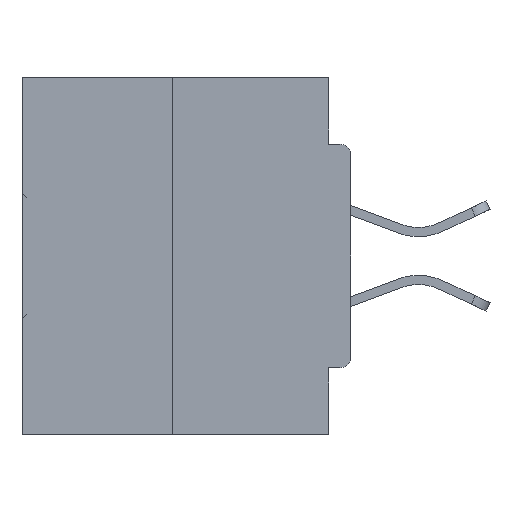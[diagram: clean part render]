
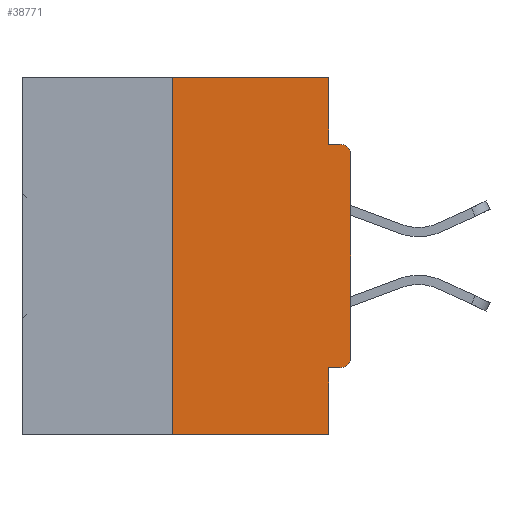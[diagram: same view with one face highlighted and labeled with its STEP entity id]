
A CAD part, left-side view. The second image highlights one B-rep face of the part: STEP entity #38771.
In plain terms, the highlighted planar face has unit normal (-1, 0, 0).
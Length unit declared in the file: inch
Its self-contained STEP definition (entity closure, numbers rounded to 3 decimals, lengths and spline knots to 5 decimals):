
#1341 = EDGE_CURVE ( 'NONE', #25626, #3799, #30260, .T. ) ;
#2344 = CARTESIAN_POINT ( 'NONE',  ( 0., 0.015, -0.4065 ) ) ;
#3655 = CIRCLE ( 'NONE', #26507, 0.015 ) ;
#3799 = VERTEX_POINT ( 'NONE', #38552 ) ;
#4048 = CARTESIAN_POINT ( 'NONE',  ( 0., 0., -0.4065 ) ) ;
#4069 = LINE ( 'NONE', #24545, #23537 ) ;
#4107 = DIRECTION ( 'NONE',  ( 0., -1., 0. ) ) ;
#4345 = DIRECTION ( 'NONE',  ( 0., 0., -1. ) ) ;
#4369 = VERTEX_POINT ( 'NONE', #11530 ) ;
#4495 = PLANE ( 'NONE',  #8993 ) ;
#4661 = DIRECTION ( 'NONE',  ( 1., 0., 0. ) ) ;
#4861 = DIRECTION ( 'NONE',  ( 0., -1., 0. ) ) ;
#5702 = LINE ( 'NONE', #25557, #31039 ) ;
#5829 = ORIENTED_EDGE ( 'NONE', *, *, #20865, .F. ) ;
#6126 = CARTESIAN_POINT ( 'NONE',  ( 0., 0.25, -0.5 ) ) ;
#6501 = VECTOR ( 'NONE', #15353, 39.37008 ) ;
#6539 = VECTOR ( 'NONE', #28233, 39.37008 ) ;
#6640 = EDGE_CURVE ( 'NONE', #15424, #7585, #7974, .T. ) ;
#7585 = VERTEX_POINT ( 'NONE', #31180 ) ;
#7686 = EDGE_CURVE ( 'NONE', #7585, #4369, #42402, .T. ) ;
#7974 = LINE ( 'NONE', #9703, #10125 ) ;
#8915 = CARTESIAN_POINT ( 'NONE',  ( 0., 0., -0.0935 ) ) ;
#8979 = ORIENTED_EDGE ( 'NONE', *, *, #30874, .T. ) ;
#8993 = AXIS2_PLACEMENT_3D ( 'NONE', #39080, #4661, #4345 ) ;
#9703 = CARTESIAN_POINT ( 'NONE',  ( 0., 0.25, 0. ) ) ;
#9841 = DIRECTION ( 'NONE',  ( 0., 0., 1. ) ) ;
#10125 = VECTOR ( 'NONE', #9841, 39.37008 ) ;
#10878 = ORIENTED_EDGE ( 'NONE', *, *, #24244, .T. ) ;
#11193 = VERTEX_POINT ( 'NONE', #11516 ) ;
#11411 = EDGE_CURVE ( 'NONE', #27176, #3799, #3655, .T. ) ;
#11516 = CARTESIAN_POINT ( 'NONE',  ( 0., 0.031, -0.5 ) ) ;
#11530 = CARTESIAN_POINT ( 'NONE',  ( 0., 0.031, 0. ) ) ;
#12800 = LINE ( 'NONE', #21237, #32812 ) ;
#13100 = DIRECTION ( 'NONE',  ( 0., 0., -1. ) ) ;
#14844 = DIRECTION ( 'NONE',  ( -1., 0., 0. ) ) ;
#14949 = ORIENTED_EDGE ( 'NONE', *, *, #30938, .F. ) ;
#15353 = DIRECTION ( 'NONE',  ( 0., 0., 1. ) ) ;
#15424 = VERTEX_POINT ( 'NONE', #6126 ) ;
#16088 = CARTESIAN_POINT ( 'NONE',  ( 0., 0., -0.3915 ) ) ;
#16958 = EDGE_CURVE ( 'NONE', #15424, #11193, #5702, .T. ) ;
#17033 = ORIENTED_EDGE ( 'NONE', *, *, #16958, .T. ) ;
#17378 = ORIENTED_EDGE ( 'NONE', *, *, #1341, .F. ) ;
#18192 = VECTOR ( 'NONE', #4107, 39.37008 ) ;
#18341 = DIRECTION ( 'NONE',  ( 0., 0., -1. ) ) ;
#18378 = ORIENTED_EDGE ( 'NONE', *, *, #7686, .F. ) ;
#18667 = EDGE_LOOP ( 'NONE', ( #18378, #20140, #17033, #32969, #5829, #8979, #10878, #19902, #17378, #14949 ) ) ;
#19902 = ORIENTED_EDGE ( 'NONE', *, *, #11411, .T. ) ;
#20140 = ORIENTED_EDGE ( 'NONE', *, *, #6640, .F. ) ;
#20865 = EDGE_CURVE ( 'NONE', #29148, #38796, #44361, .T. ) ;
#21237 = CARTESIAN_POINT ( 'NONE',  ( 0., 0.031, 0. ) ) ;
#21990 = CIRCLE ( 'NONE', #40048, 0.015 ) ;
#23537 = VECTOR ( 'NONE', #28024, 39.37008 ) ;
#24244 = EDGE_CURVE ( 'NONE', #26953, #27176, #27032, .T. ) ;
#24396 = FACE_OUTER_BOUND ( 'NONE', #18667, .T. ) ;
#24545 = CARTESIAN_POINT ( 'NONE',  ( 0., 0.031, -0.5 ) ) ;
#25557 = CARTESIAN_POINT ( 'NONE',  ( 0., 0.46, -0.5 ) ) ;
#25626 = VERTEX_POINT ( 'NONE', #39213 ) ;
#25875 = DIRECTION ( 'NONE',  ( 0., -1., 0. ) ) ;
#26507 = AXIS2_PLACEMENT_3D ( 'NONE', #28308, #14844, #18341 ) ;
#26953 = VERTEX_POINT ( 'NONE', #16088 ) ;
#27032 = LINE ( 'NONE', #35912, #6501 ) ;
#27176 = VERTEX_POINT ( 'NONE', #42749 ) ;
#28024 = DIRECTION ( 'NONE',  ( 0., 0., -1. ) ) ;
#28233 = DIRECTION ( 'NONE',  ( 0., 1., 0. ) ) ;
#28308 = CARTESIAN_POINT ( 'NONE',  ( 0., 0.015, -0.1085 ) ) ;
#29148 = VERTEX_POINT ( 'NONE', #2344 ) ;
#30260 = LINE ( 'NONE', #8915, #41554 ) ;
#30492 = CARTESIAN_POINT ( 'NONE',  ( 0., 0.015, -0.3915 ) ) ;
#30874 = EDGE_CURVE ( 'NONE', #29148, #26953, #21990, .T. ) ;
#30938 = EDGE_CURVE ( 'NONE', #4369, #25626, #12800, .T. ) ;
#31039 = VECTOR ( 'NONE', #25875, 39.37008 ) ;
#31180 = CARTESIAN_POINT ( 'NONE',  ( 0., 0.25, 0. ) ) ;
#32812 = VECTOR ( 'NONE', #38604, 39.37008 ) ;
#32969 = ORIENTED_EDGE ( 'NONE', *, *, #36851, .F. ) ;
#33822 = DIRECTION ( 'NONE',  ( -1., 0., 0. ) ) ;
#35545 = CARTESIAN_POINT ( 'NONE',  ( 0., 0.46, 0. ) ) ;
#35912 = CARTESIAN_POINT ( 'NONE',  ( 0., 0., 0. ) ) ;
#36851 = EDGE_CURVE ( 'NONE', #38796, #11193, #4069, .T. ) ;
#38552 = CARTESIAN_POINT ( 'NONE',  ( 0., 0.015, -0.0935 ) ) ;
#38604 = DIRECTION ( 'NONE',  ( 0., 0., -1. ) ) ;
#38771 = ADVANCED_FACE ( 'NONE', ( #24396 ), #4495, .F. ) ;
#38796 = VERTEX_POINT ( 'NONE', #42534 ) ;
#39080 = CARTESIAN_POINT ( 'NONE',  ( 0., 0.46, 0. ) ) ;
#39213 = CARTESIAN_POINT ( 'NONE',  ( 0., 0.031, -0.0935 ) ) ;
#40048 = AXIS2_PLACEMENT_3D ( 'NONE', #30492, #33822, #13100 ) ;
#41554 = VECTOR ( 'NONE', #4861, 39.37008 ) ;
#42402 = LINE ( 'NONE', #35545, #18192 ) ;
#42534 = CARTESIAN_POINT ( 'NONE',  ( 0., 0.031, -0.4065 ) ) ;
#42749 = CARTESIAN_POINT ( 'NONE',  ( 0., 0., -0.1085 ) ) ;
#44361 = LINE ( 'NONE', #4048, #6539 ) ;
